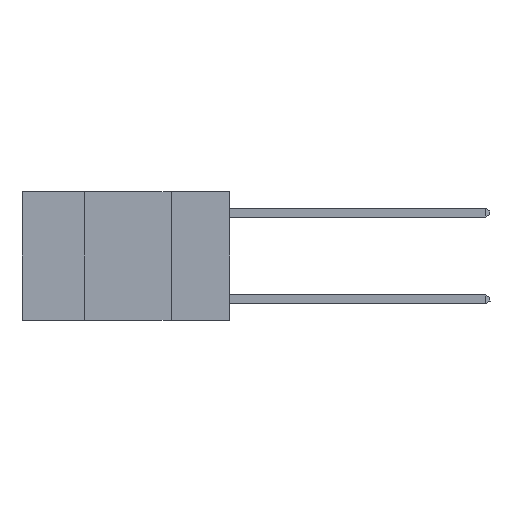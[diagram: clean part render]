
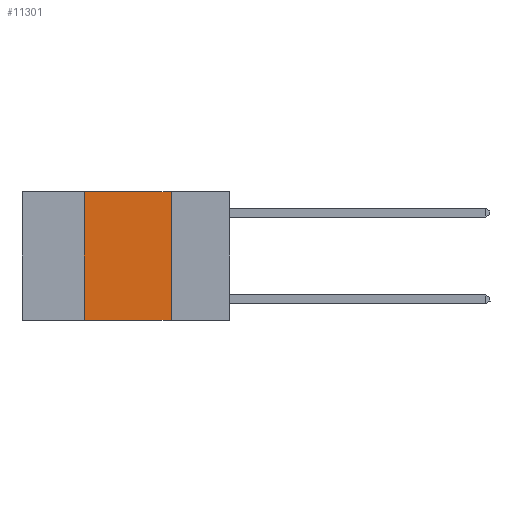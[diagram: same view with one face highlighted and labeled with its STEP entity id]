
A CAD part, left-side view. The second image highlights one B-rep face of the part: STEP entity #11301.
In plain terms, the highlighted planar face has unit normal (-1, 0, 0).
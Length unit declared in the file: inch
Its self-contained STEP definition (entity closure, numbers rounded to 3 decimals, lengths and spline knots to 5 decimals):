
#755 = CARTESIAN_POINT ( 'NONE',  ( 0., 0.6, 0. ) ) ;
#779 = VERTEX_POINT ( 'NONE', #7380 ) ;
#1040 = LINE ( 'NONE', #10882, #14788 ) ;
#1542 = EDGE_CURVE ( 'NONE', #8707, #8510, #16136, .T. ) ;
#2172 = VECTOR ( 'NONE', #3903, 39.37008 ) ;
#3886 = FACE_OUTER_BOUND ( 'NONE', #4679, .T. ) ;
#3903 = DIRECTION ( 'NONE',  ( 0., -1., 0. ) ) ;
#4679 = EDGE_LOOP ( 'NONE', ( #10379, #14154, #10823, #13799 ) ) ;
#5117 = PLANE ( 'NONE',  #8132 ) ;
#5477 = CARTESIAN_POINT ( 'NONE',  ( 0., 0.17, 0. ) ) ;
#7380 = CARTESIAN_POINT ( 'NONE',  ( 0., 0.42, 0. ) ) ;
#7636 = LINE ( 'NONE', #755, #11502 ) ;
#8011 = DIRECTION ( 'NONE',  ( 0., 0., -1. ) ) ;
#8132 = AXIS2_PLACEMENT_3D ( 'NONE', #15121, #16514, #8011 ) ;
#8370 = DIRECTION ( 'NONE',  ( 0., 0., -1. ) ) ;
#8510 = VERTEX_POINT ( 'NONE', #17600 ) ;
#8707 = VERTEX_POINT ( 'NONE', #9606 ) ;
#9109 = VERTEX_POINT ( 'NONE', #17640 ) ;
#9606 = CARTESIAN_POINT ( 'NONE',  ( 0., 0.17, 0. ) ) ;
#10379 = ORIENTED_EDGE ( 'NONE', *, *, #1542, .F. ) ;
#10667 = DIRECTION ( 'NONE',  ( 0., -1., 0. ) ) ;
#10823 = ORIENTED_EDGE ( 'NONE', *, *, #16906, .F. ) ;
#10882 = CARTESIAN_POINT ( 'NONE',  ( 0., 0.42, 0. ) ) ;
#11097 = CARTESIAN_POINT ( 'NONE',  ( 0., 0.6, -0.37 ) ) ;
#11301 = ADVANCED_FACE ( 'NONE', ( #3886 ), #5117, .F. ) ;
#11502 = VECTOR ( 'NONE', #10667, 39.37008 ) ;
#12354 = DIRECTION ( 'NONE',  ( 0., 0., 1. ) ) ;
#12449 = EDGE_CURVE ( 'NONE', #779, #8707, #7636, .T. ) ;
#12458 = VECTOR ( 'NONE', #8370, 39.37008 ) ;
#13546 = LINE ( 'NONE', #11097, #2172 ) ;
#13799 = ORIENTED_EDGE ( 'NONE', *, *, #14999, .T. ) ;
#14154 = ORIENTED_EDGE ( 'NONE', *, *, #12449, .F. ) ;
#14788 = VECTOR ( 'NONE', #12354, 39.37008 ) ;
#14999 = EDGE_CURVE ( 'NONE', #9109, #8510, #13546, .T. ) ;
#15121 = CARTESIAN_POINT ( 'NONE',  ( 0., 0.6, 0. ) ) ;
#16136 = LINE ( 'NONE', #5477, #12458 ) ;
#16514 = DIRECTION ( 'NONE',  ( 1., 0., 0. ) ) ;
#16906 = EDGE_CURVE ( 'NONE', #9109, #779, #1040, .T. ) ;
#17600 = CARTESIAN_POINT ( 'NONE',  ( 0., 0.17, -0.37 ) ) ;
#17640 = CARTESIAN_POINT ( 'NONE',  ( 0., 0.42, -0.37 ) ) ;
